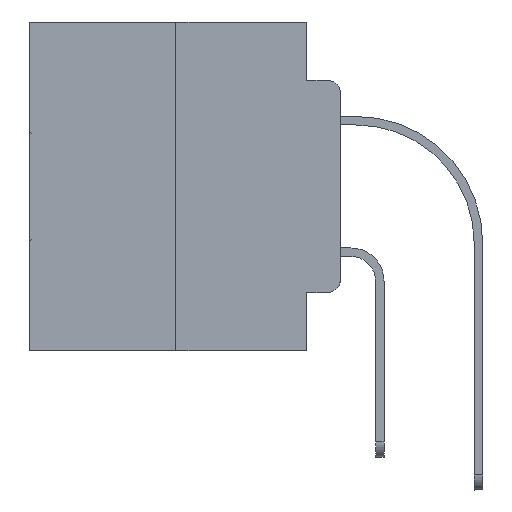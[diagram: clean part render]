
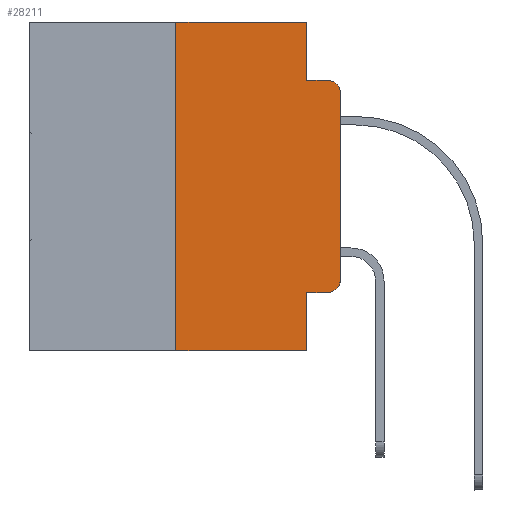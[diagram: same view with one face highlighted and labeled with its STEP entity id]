
A CAD part, left-side view. The second image highlights one B-rep face of the part: STEP entity #28211.
In plain terms, the highlighted planar face has unit normal (-1, 0, 0).
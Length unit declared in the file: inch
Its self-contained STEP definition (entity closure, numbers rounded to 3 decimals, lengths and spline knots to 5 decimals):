
#530 = ORIENTED_EDGE ( 'NONE', *, *, #19289, .F. ) ;
#593 = CARTESIAN_POINT ( 'NONE',  ( 0., 0.051, 0. ) ) ;
#1596 = VERTEX_POINT ( 'NONE', #27613 ) ;
#1963 = VERTEX_POINT ( 'NONE', #593 ) ;
#1989 = CIRCLE ( 'NONE', #25628, 0.02 ) ;
#2018 = EDGE_LOOP ( 'NONE', ( #21536, #22502, #25337, #530, #18310, #5918, #29847, #26884, #11125, #25980 ) ) ;
#2900 = VECTOR ( 'NONE', #17602, 39.37008 ) ;
#3172 = LINE ( 'NONE', #17693, #29023 ) ;
#3893 = EDGE_CURVE ( 'NONE', #6554, #1596, #3172, .T. ) ;
#4184 = PLANE ( 'NONE',  #7554 ) ;
#4379 = CARTESIAN_POINT ( 'NONE',  ( 0., 0., -0.3915 ) ) ;
#5249 = DIRECTION ( 'NONE',  ( 0., -1., 0. ) ) ;
#5918 = ORIENTED_EDGE ( 'NONE', *, *, #26329, .F. ) ;
#6082 = CARTESIAN_POINT ( 'NONE',  ( 0., 0.473, 0. ) ) ;
#6125 = EDGE_CURVE ( 'NONE', #30947, #1963, #10224, .T. ) ;
#6130 = CARTESIAN_POINT ( 'NONE',  ( 0., 0.25, 0. ) ) ;
#6132 = CARTESIAN_POINT ( 'NONE',  ( 0., 0., 0. ) ) ;
#6346 = DIRECTION ( 'NONE',  ( -1., 0., 0. ) ) ;
#6554 = VERTEX_POINT ( 'NONE', #17420 ) ;
#7153 = DIRECTION ( 'NONE',  ( 0., -1., 0. ) ) ;
#7426 = DIRECTION ( 'NONE',  ( 0., -1., 0. ) ) ;
#7554 = AXIS2_PLACEMENT_3D ( 'NONE', #6082, #15695, #27992 ) ;
#7731 = CARTESIAN_POINT ( 'NONE',  ( 0., 0.051, -0.4115 ) ) ;
#8627 = VECTOR ( 'NONE', #7153, 39.37008 ) ;
#10224 = LINE ( 'NONE', #19820, #27651 ) ;
#10584 = DIRECTION ( 'NONE',  ( -1., 0., 0. ) ) ;
#10859 = CARTESIAN_POINT ( 'NONE',  ( 0., 0., -0.1085 ) ) ;
#10915 = DIRECTION ( 'NONE',  ( 0., 0., -1. ) ) ;
#11125 = ORIENTED_EDGE ( 'NONE', *, *, #16552, .T. ) ;
#11386 = EDGE_CURVE ( 'NONE', #29175, #14423, #23130, .T. ) ;
#11413 = CIRCLE ( 'NONE', #15425, 0.02 ) ;
#12583 = EDGE_CURVE ( 'NONE', #24923, #19781, #14707, .T. ) ;
#12629 = LINE ( 'NONE', #22232, #19890 ) ;
#14423 = VERTEX_POINT ( 'NONE', #10859 ) ;
#14707 = LINE ( 'NONE', #24297, #8627 ) ;
#15425 = AXIS2_PLACEMENT_3D ( 'NONE', #17995, #6346, #10915 ) ;
#15452 = DIRECTION ( 'NONE',  ( 0., 0., -1. ) ) ;
#15695 = DIRECTION ( 'NONE',  ( 1., 0., 0. ) ) ;
#16291 = CARTESIAN_POINT ( 'NONE',  ( 0., 0.02, -0.4115 ) ) ;
#16552 = EDGE_CURVE ( 'NONE', #29768, #30110, #29034, .T. ) ;
#16806 = VECTOR ( 'NONE', #7426, 39.37008 ) ;
#17420 = CARTESIAN_POINT ( 'NONE',  ( 0., 0.25, -0.5 ) ) ;
#17460 = LINE ( 'NONE', #19517, #21872 ) ;
#17602 = DIRECTION ( 'NONE',  ( 0., 0., 1. ) ) ;
#17693 = CARTESIAN_POINT ( 'NONE',  ( 0., 0.473, -0.5 ) ) ;
#17995 = CARTESIAN_POINT ( 'NONE',  ( 0., 0.02, -0.1085 ) ) ;
#18310 = ORIENTED_EDGE ( 'NONE', *, *, #6125, .F. ) ;
#18315 = EDGE_CURVE ( 'NONE', #29768, #1596, #17460, .T. ) ;
#18516 = FACE_OUTER_BOUND ( 'NONE', #2018, .T. ) ;
#19289 = EDGE_CURVE ( 'NONE', #1963, #24923, #12629, .T. ) ;
#19517 = CARTESIAN_POINT ( 'NONE',  ( 0., 0.051, 0. ) ) ;
#19684 = DIRECTION ( 'NONE',  ( 0., 0., -1. ) ) ;
#19781 = VERTEX_POINT ( 'NONE', #21021 ) ;
#19820 = CARTESIAN_POINT ( 'NONE',  ( 0., 0.473, 0. ) ) ;
#19890 = VECTOR ( 'NONE', #15452, 39.37008 ) ;
#20013 = EDGE_CURVE ( 'NONE', #14423, #19781, #11413, .T. ) ;
#20606 = DIRECTION ( 'NONE',  ( 0., 0., 1. ) ) ;
#21021 = CARTESIAN_POINT ( 'NONE',  ( 0., 0.02, -0.0885 ) ) ;
#21536 = ORIENTED_EDGE ( 'NONE', *, *, #11386, .T. ) ;
#21658 = CARTESIAN_POINT ( 'NONE',  ( 0., 0.051, -0.4115 ) ) ;
#21848 = CARTESIAN_POINT ( 'NONE',  ( 0., 0.051, -0.0885 ) ) ;
#21872 = VECTOR ( 'NONE', #19684, 39.37008 ) ;
#22232 = CARTESIAN_POINT ( 'NONE',  ( 0., 0.051, 0. ) ) ;
#22502 = ORIENTED_EDGE ( 'NONE', *, *, #20013, .T. ) ;
#22958 = DIRECTION ( 'NONE',  ( 0., -1., 0. ) ) ;
#23130 = LINE ( 'NONE', #6132, #24663 ) ;
#24251 = EDGE_CURVE ( 'NONE', #30110, #29175, #1989, .T. ) ;
#24297 = CARTESIAN_POINT ( 'NONE',  ( 0., 0.051, -0.0885 ) ) ;
#24663 = VECTOR ( 'NONE', #20606, 39.37008 ) ;
#24828 = CARTESIAN_POINT ( 'NONE',  ( 0., 0.25, 0. ) ) ;
#24923 = VERTEX_POINT ( 'NONE', #21848 ) ;
#25051 = CARTESIAN_POINT ( 'NONE',  ( 0., 0.02, -0.3915 ) ) ;
#25337 = ORIENTED_EDGE ( 'NONE', *, *, #12583, .F. ) ;
#25628 = AXIS2_PLACEMENT_3D ( 'NONE', #25051, #10584, #29822 ) ;
#25980 = ORIENTED_EDGE ( 'NONE', *, *, #24251, .T. ) ;
#26329 = EDGE_CURVE ( 'NONE', #6554, #30947, #29288, .T. ) ;
#26884 = ORIENTED_EDGE ( 'NONE', *, *, #18315, .F. ) ;
#27613 = CARTESIAN_POINT ( 'NONE',  ( 0., 0.051, -0.5 ) ) ;
#27651 = VECTOR ( 'NONE', #22958, 39.37008 ) ;
#27992 = DIRECTION ( 'NONE',  ( 0., 0., -1. ) ) ;
#28211 = ADVANCED_FACE ( 'NONE', ( #18516 ), #4184, .F. ) ;
#29023 = VECTOR ( 'NONE', #5249, 39.37008 ) ;
#29034 = LINE ( 'NONE', #7731, #16806 ) ;
#29175 = VERTEX_POINT ( 'NONE', #4379 ) ;
#29288 = LINE ( 'NONE', #24828, #2900 ) ;
#29768 = VERTEX_POINT ( 'NONE', #21658 ) ;
#29822 = DIRECTION ( 'NONE',  ( 0., 0., -1. ) ) ;
#29847 = ORIENTED_EDGE ( 'NONE', *, *, #3893, .T. ) ;
#30110 = VERTEX_POINT ( 'NONE', #16291 ) ;
#30947 = VERTEX_POINT ( 'NONE', #6130 ) ;
